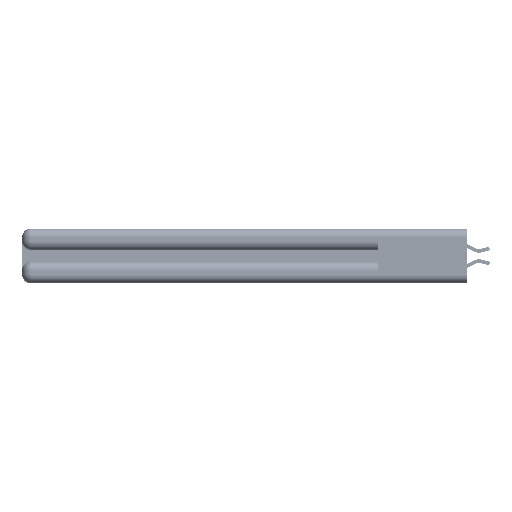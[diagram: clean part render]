
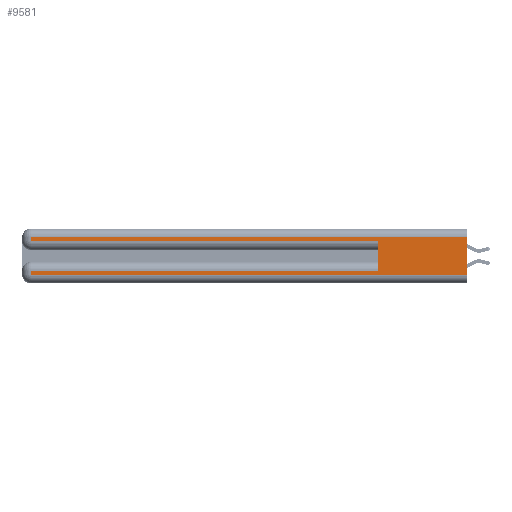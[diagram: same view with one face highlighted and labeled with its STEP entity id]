
A CAD part, left-side view. The second image highlights one B-rep face of the part: STEP entity #9581.
In plain terms, the highlighted planar face has unit normal (-1, 0, 0).
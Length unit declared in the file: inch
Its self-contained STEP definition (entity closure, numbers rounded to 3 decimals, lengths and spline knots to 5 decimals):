
#1365 = CARTESIAN_POINT ( 'NONE',  ( 0., 2.94, 0.285 ) ) ;
#2006 = ORIENTED_EDGE ( 'NONE', *, *, #30893, .F. ) ;
#2125 = VECTOR ( 'NONE', #25412, 39.37008 ) ;
#2318 = ORIENTED_EDGE ( 'NONE', *, *, #29446, .T. ) ;
#3229 = EDGE_CURVE ( 'NONE', #17608, #8873, #30942, .T. ) ;
#4156 = CARTESIAN_POINT ( 'NONE',  ( 0., 0., 0.37 ) ) ;
#5537 = EDGE_CURVE ( 'NONE', #24533, #19931, #49792, .T. ) ;
#6319 = ORIENTED_EDGE ( 'NONE', *, *, #3229, .T. ) ;
#6759 = LINE ( 'NONE', #23428, #47719 ) ;
#7150 = CARTESIAN_POINT ( 'NONE',  ( 0., 0., 0.37 ) ) ;
#8163 = DIRECTION ( 'NONE',  ( 1., 0., 0. ) ) ;
#8711 = VECTOR ( 'NONE', #34933, 39.37008 ) ;
#8873 = VERTEX_POINT ( 'NONE', #31449 ) ;
#8900 = CARTESIAN_POINT ( 'NONE',  ( 0., 0.6, 0.085 ) ) ;
#9581 = ADVANCED_FACE ( 'NONE', ( #49348 ), #27928, .F. ) ;
#10105 = LINE ( 'NONE', #30385, #51003 ) ;
#12019 = CARTESIAN_POINT ( 'NONE',  ( 0., 2.94, 0.37 ) ) ;
#13369 = ORIENTED_EDGE ( 'NONE', *, *, #40295, .T. ) ;
#14787 = DIRECTION ( 'NONE',  ( 0., 0., -1. ) ) ;
#16859 = DIRECTION ( 'NONE',  ( 0., 0., 1. ) ) ;
#16971 = VERTEX_POINT ( 'NONE', #1365 ) ;
#17608 = VERTEX_POINT ( 'NONE', #41541 ) ;
#18408 = DIRECTION ( 'NONE',  ( 0., -1., 0. ) ) ;
#18587 = VERTEX_POINT ( 'NONE', #31081 ) ;
#18690 = EDGE_CURVE ( 'NONE', #8873, #16971, #19917, .T. ) ;
#18872 = VECTOR ( 'NONE', #14787, 39.37008 ) ;
#18937 = CARTESIAN_POINT ( 'NONE',  ( 0., 2.94, 0.085 ) ) ;
#19240 = LINE ( 'NONE', #7150, #8711 ) ;
#19796 = CARTESIAN_POINT ( 'NONE',  ( 0., 0., 0.31 ) ) ;
#19917 = LINE ( 'NONE', #12019, #29220 ) ;
#19931 = VERTEX_POINT ( 'NONE', #50705 ) ;
#19970 = DIRECTION ( 'NONE',  ( 0., 0., -1. ) ) ;
#21421 = CARTESIAN_POINT ( 'NONE',  ( 0., 0., 0.085 ) ) ;
#23428 = CARTESIAN_POINT ( 'NONE',  ( 0., 0., 0.285 ) ) ;
#24533 = VERTEX_POINT ( 'NONE', #8900 ) ;
#25412 = DIRECTION ( 'NONE',  ( 0., 1., 0. ) ) ;
#26227 = VECTOR ( 'NONE', #16859, 39.37008 ) ;
#27551 = ORIENTED_EDGE ( 'NONE', *, *, #32363, .T. ) ;
#27928 = PLANE ( 'NONE',  #28266 ) ;
#28266 = AXIS2_PLACEMENT_3D ( 'NONE', #4156, #8163, #35917 ) ;
#29220 = VECTOR ( 'NONE', #19970, 39.37008 ) ;
#29446 = EDGE_CURVE ( 'NONE', #32459, #18587, #10105, .T. ) ;
#29748 = ORIENTED_EDGE ( 'NONE', *, *, #5537, .F. ) ;
#30385 = CARTESIAN_POINT ( 'NONE',  ( 0., 0., 0.06 ) ) ;
#30893 = EDGE_CURVE ( 'NONE', #17608, #18587, #19240, .T. ) ;
#30942 = LINE ( 'NONE', #19796, #41455 ) ;
#31081 = CARTESIAN_POINT ( 'NONE',  ( 0., 0., 0.06 ) ) ;
#31449 = CARTESIAN_POINT ( 'NONE',  ( 0., 2.94, 0.31 ) ) ;
#32363 = EDGE_CURVE ( 'NONE', #16971, #19931, #6759, .T. ) ;
#32459 = VERTEX_POINT ( 'NONE', #47498 ) ;
#33816 = LINE ( 'NONE', #21421, #2125 ) ;
#34549 = CARTESIAN_POINT ( 'NONE',  ( 0., 2.94, 0.37 ) ) ;
#34933 = DIRECTION ( 'NONE',  ( 0., 0., -1. ) ) ;
#35917 = DIRECTION ( 'NONE',  ( 0., 0., -1. ) ) ;
#36622 = CARTESIAN_POINT ( 'NONE',  ( 0., 0.6, 0.145 ) ) ;
#39961 = LINE ( 'NONE', #34549, #18872 ) ;
#40295 = EDGE_CURVE ( 'NONE', #50742, #32459, #39961, .T. ) ;
#41455 = VECTOR ( 'NONE', #47519, 39.37008 ) ;
#41541 = CARTESIAN_POINT ( 'NONE',  ( 0., 0., 0.31 ) ) ;
#41621 = EDGE_LOOP ( 'NONE', ( #2006, #6319, #46978, #27551, #29748, #41893, #13369, #2318 ) ) ;
#41893 = ORIENTED_EDGE ( 'NONE', *, *, #43516, .T. ) ;
#43516 = EDGE_CURVE ( 'NONE', #24533, #50742, #33816, .T. ) ;
#46978 = ORIENTED_EDGE ( 'NONE', *, *, #18690, .T. ) ;
#47498 = CARTESIAN_POINT ( 'NONE',  ( 0., 2.94, 0.06 ) ) ;
#47519 = DIRECTION ( 'NONE',  ( 0., 1., 0. ) ) ;
#47719 = VECTOR ( 'NONE', #51137, 39.37008 ) ;
#49348 = FACE_OUTER_BOUND ( 'NONE', #41621, .T. ) ;
#49792 = LINE ( 'NONE', #36622, #26227 ) ;
#50705 = CARTESIAN_POINT ( 'NONE',  ( 0., 0.6, 0.285 ) ) ;
#50742 = VERTEX_POINT ( 'NONE', #18937 ) ;
#51003 = VECTOR ( 'NONE', #18408, 39.37008 ) ;
#51137 = DIRECTION ( 'NONE',  ( 0., -1., 0. ) ) ;
